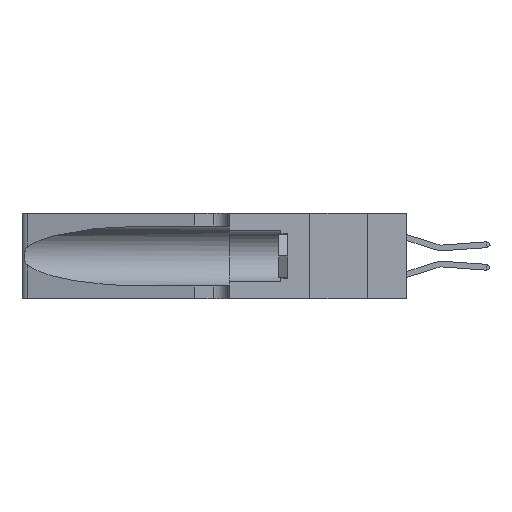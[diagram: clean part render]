
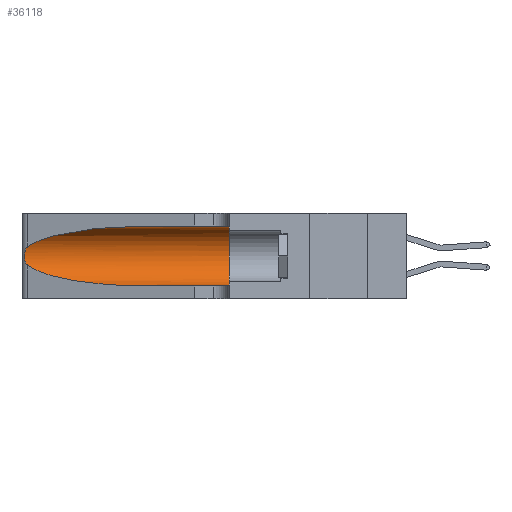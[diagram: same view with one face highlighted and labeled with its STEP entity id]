
A CAD part, left-side view. The second image highlights one B-rep face of the part: STEP entity #36118.
In plain terms, the highlighted cylindrical face has radius 3.308 mm (diameter 6.617 mm), a partial arc.
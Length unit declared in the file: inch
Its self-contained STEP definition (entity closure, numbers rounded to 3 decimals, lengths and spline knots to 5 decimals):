
#697 = ORIENTED_EDGE ( 'NONE', *, *, #2098, .T. ) ;
#909 = CARTESIAN_POINT ( 'NONE',  ( 0.25854, 1.2359, 0.20912 ) ) ;
#1372 = CARTESIAN_POINT ( 'NONE',  ( 0.26017, 1.23833, 0.17102 ) ) ;
#1463 = B_SPLINE_CURVE_WITH_KNOTS ( 'NONE', 3,
 ( #3820, #28157, #25589, #4735, #909, #22088, #32243, #14923, #1372, #21779, #14768, #25283, #25430, #42922 ),
 .UNSPECIFIED., .F., .F.,
 ( 4, 2, 2, 2, 2, 2, 4 ),
 ( 0., 0.00027, 0.00053, 0.00107, 0.0016, 0.00187, 0.00214 ),
 .UNSPECIFIED. ) ;
#1803 = CARTESIAN_POINT ( 'NONE',  ( 0.1305, 0.35, 0.05475 ) ) ;
#2098 = EDGE_CURVE ( 'NONE', #17165, #31821, #6600, .T. ) ;
#2233 = DIRECTION ( 'NONE',  ( 0., -1., 0. ) ) ;
#2914 = CARTESIAN_POINT ( 'NONE',  ( 0.18966, 0.96281, 0.05475 ) ) ;
#3234 = DIRECTION ( 'NONE',  ( 0., 0., 1. ) ) ;
#3820 = CARTESIAN_POINT ( 'NONE',  ( 0.25487, 1.22718, 0.22369 ) ) ;
#4735 = CARTESIAN_POINT ( 'NONE',  ( 0.25787, 1.23484, 0.2124 ) ) ;
#5441 = VERTEX_POINT ( 'NONE', #15443 ) ;
#6600 = LINE ( 'NONE', #35283, #8206 ) ;
#7007 = CARTESIAN_POINT ( 'NONE',  ( 0.25487, 1.22718, 0.22369 ) ) ;
#7564 = DIRECTION ( 'NONE',  ( 0., -1., 0. ) ) ;
#8206 = VECTOR ( 'NONE', #7564, 39.37008 ) ;
#8220 = VERTEX_POINT ( 'NONE', #27672 ) ;
#8267 = CARTESIAN_POINT ( 'NONE',  ( 0.1305, 1.61858, 0.31525 ) ) ;
#11655 = DIRECTION ( 'NONE',  ( 0., -1., 0. ) ) ;
#12760 = ORIENTED_EDGE ( 'NONE', *, *, #21962, .T. ) ;
#13016 = CARTESIAN_POINT ( 'NONE',  ( 0.1305, 0.72297, 0.05475 ) ) ;
#13294 = DIRECTION ( 'NONE',  ( 0., 1., 0. ) ) ;
#14768 = CARTESIAN_POINT ( 'NONE',  ( 0.25789, 1.23486, 0.15765 ) ) ;
#14923 = CARTESIAN_POINT ( 'NONE',  ( 0.26075, 1.23896, 0.178 ) ) ;
#15316 = ORIENTED_EDGE ( 'NONE', *, *, #35117, .T. ) ;
#15443 = CARTESIAN_POINT ( 'NONE',  ( 0.1305, 0.72297, 0.31525 ) ) ;
#16267 = EDGE_LOOP ( 'NONE', ( #24509, #15316, #12760, #697, #19594, #21987 ) ) ;
#17058 = CARTESIAN_POINT ( 'NONE',  ( 0.25487, 1.22718, 0.14631 ) ) ;
#17165 = VERTEX_POINT ( 'NONE', #13016 ) ;
#18346 = CARTESIAN_POINT ( 'NONE',  ( 0.1305, 0.35, 0.31525 ) ) ;
#19137 = DIRECTION ( 'NONE',  ( 0., 0., -1. ) ) ;
#19594 = ORIENTED_EDGE ( 'NONE', *, *, #40558, .F. ) ;
#19761 = AXIS2_PLACEMENT_3D ( 'NONE', #34113, #13294, #3234 ) ;
#20909 = CARTESIAN_POINT ( 'NONE',  ( 0.2373, 1.15595, 0.28018 ) ) ;
#21355 = FACE_OUTER_BOUND ( 'NONE', #16267, .T. ) ;
#21779 = CARTESIAN_POINT ( 'NONE',  ( 0.25856, 1.23593, 0.16098 ) ) ;
#21962 = EDGE_CURVE ( 'NONE', #26062, #17165, #42741, .T. ) ;
#21987 = ORIENTED_EDGE ( 'NONE', *, *, #28092, .F. ) ;
#22088 = CARTESIAN_POINT ( 'NONE',  ( 0.26018, 1.23835, 0.19895 ) ) ;
#24251 = CARTESIAN_POINT ( 'NONE',  ( 0.18966, 0.96281, 0.31525 ) ) ;
#24509 = ORIENTED_EDGE ( 'NONE', *, *, #28585, .T. ) ;
#24942 = CIRCLE ( 'NONE', #19761, 0.13025 ) ;
#25283 = CARTESIAN_POINT ( 'NONE',  ( 0.25639, 1.23186, 0.15144 ) ) ;
#25430 = CARTESIAN_POINT ( 'NONE',  ( 0.25555, 1.22993, 0.14849 ) ) ;
#25589 = CARTESIAN_POINT ( 'NONE',  ( 0.25639, 1.23184, 0.21858 ) ) ;
#25755 =( BOUNDED_CURVE ( )  B_SPLINE_CURVE ( 3, ( #41615, #24251, #20909, #7007 ),
 .UNSPECIFIED., .F., .F. ) 
 B_SPLINE_CURVE_WITH_KNOTS ( ( 4, 4 ),
 ( 1.5708, 2.84003 ),
 .UNSPECIFIED. ) 
 CURVE ( )  GEOMETRIC_REPRESENTATION_ITEM ( )  RATIONAL_B_SPLINE_CURVE ( ( 1., 0.87, 0.87, 1. ) ) 
 REPRESENTATION_ITEM ( '' )  );
#26062 = VERTEX_POINT ( 'NONE', #17058 ) ;
#27672 = CARTESIAN_POINT ( 'NONE',  ( 0.25487, 1.22718, 0.22369 ) ) ;
#28092 = EDGE_CURVE ( 'NONE', #5441, #42164, #35280, .T. ) ;
#28157 = CARTESIAN_POINT ( 'NONE',  ( 0.25555, 1.22994, 0.2215 ) ) ;
#28585 = EDGE_CURVE ( 'NONE', #5441, #8220, #25755, .T. ) ;
#28732 = VECTOR ( 'NONE', #11655, 39.37008 ) ;
#31821 = VERTEX_POINT ( 'NONE', #1803 ) ;
#32243 = CARTESIAN_POINT ( 'NONE',  ( 0.26075, 1.23896, 0.19203 ) ) ;
#33296 = CYLINDRICAL_SURFACE ( 'NONE', #37591, 0.13025 ) ;
#34113 = CARTESIAN_POINT ( 'NONE',  ( 0.1305, 0.35, 0.185 ) ) ;
#35117 = EDGE_CURVE ( 'NONE', #8220, #26062, #1463, .T. ) ;
#35280 = LINE ( 'NONE', #8267, #28732 ) ;
#35283 = CARTESIAN_POINT ( 'NONE',  ( 0.1305, 1.61858, 0.05475 ) ) ;
#36118 = ADVANCED_FACE ( 'NONE', ( #21355 ), #33296, .F. ) ;
#36922 = CARTESIAN_POINT ( 'NONE',  ( 0.1305, 1.61858, 0.185 ) ) ;
#37591 = AXIS2_PLACEMENT_3D ( 'NONE', #36922, #2233, #19137 ) ;
#37612 = CARTESIAN_POINT ( 'NONE',  ( 0.2373, 1.15595, 0.08982 ) ) ;
#40558 = EDGE_CURVE ( 'NONE', #42164, #31821, #24942, .T. ) ;
#41114 = CARTESIAN_POINT ( 'NONE',  ( 0.1305, 0.72297, 0.05475 ) ) ;
#41261 = CARTESIAN_POINT ( 'NONE',  ( 0.25487, 1.22718, 0.14631 ) ) ;
#41615 = CARTESIAN_POINT ( 'NONE',  ( 0.1305, 0.72297, 0.31525 ) ) ;
#42164 = VERTEX_POINT ( 'NONE', #18346 ) ;
#42741 =( BOUNDED_CURVE ( )  B_SPLINE_CURVE ( 3, ( #41261, #37612, #2914, #41114 ),
 .UNSPECIFIED., .F., .F. ) 
 B_SPLINE_CURVE_WITH_KNOTS ( ( 4, 4 ),
 ( 3.44316, 4.71239 ),
 .UNSPECIFIED. ) 
 CURVE ( )  GEOMETRIC_REPRESENTATION_ITEM ( )  RATIONAL_B_SPLINE_CURVE ( ( 1., 0.87, 0.87, 1. ) ) 
 REPRESENTATION_ITEM ( '' )  );
#42922 = CARTESIAN_POINT ( 'NONE',  ( 0.25487, 1.22718, 0.14631 ) ) ;
